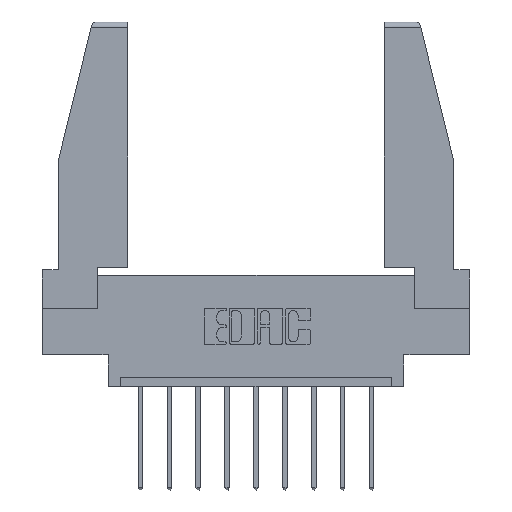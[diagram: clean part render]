
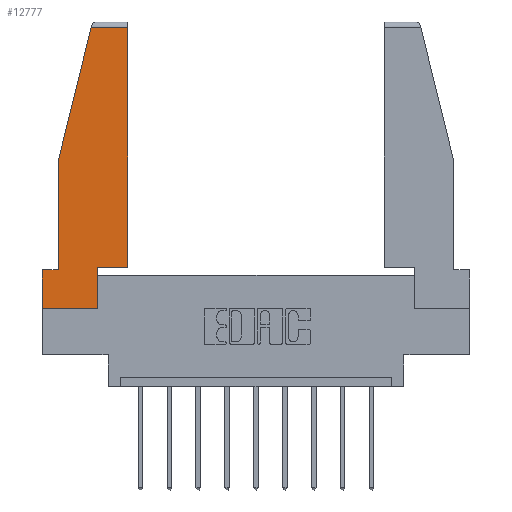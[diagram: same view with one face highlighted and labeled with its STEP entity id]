
A CAD part, top view. The second image highlights one B-rep face of the part: STEP entity #12777.
In plain terms, the highlighted planar face has unit normal (0, 0, 1).
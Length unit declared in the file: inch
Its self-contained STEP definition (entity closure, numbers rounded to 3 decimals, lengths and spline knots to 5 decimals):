
#294 = VECTOR ( 'NONE', #7641, 39.37008 ) ;
#522 = VECTOR ( 'NONE', #7283, 39.37008 ) ;
#584 = VERTEX_POINT ( 'NONE', #11970 ) ;
#839 = CARTESIAN_POINT ( 'NONE',  ( 0., 0.21, 0. ) ) ;
#1178 = DIRECTION ( 'NONE',  ( 1., 0., 0. ) ) ;
#1516 = EDGE_CURVE ( 'NONE', #584, #4535, #6369, .T. ) ;
#1833 = ORIENTED_EDGE ( 'NONE', *, *, #11407, .T. ) ;
#1986 = ORIENTED_EDGE ( 'NONE', *, *, #10798, .T. ) ;
#1992 = EDGE_CURVE ( 'NONE', #4535, #5249, #11923, .T. ) ;
#1998 = CARTESIAN_POINT ( 'NONE',  ( 0.2636, 1.52, 0. ) ) ;
#2097 = EDGE_LOOP ( 'NONE', ( #1986, #8258, #13383, #1833, #10948, #2662, #8005, #8778, #3963 ) ) ;
#2192 = LINE ( 'NONE', #2314, #13155 ) ;
#2307 = LINE ( 'NONE', #11112, #522 ) ;
#2314 = CARTESIAN_POINT ( 'NONE',  ( 0., 0., 0. ) ) ;
#2662 = ORIENTED_EDGE ( 'NONE', *, *, #1992, .T. ) ;
#2899 = VECTOR ( 'NONE', #10846, 39.37008 ) ;
#3237 = EDGE_CURVE ( 'NONE', #8121, #9064, #6634, .T. ) ;
#3409 = EDGE_CURVE ( 'NONE', #4603, #11067, #10568, .T. ) ;
#3734 = VERTEX_POINT ( 'NONE', #4488 ) ;
#3735 = LINE ( 'NONE', #11987, #2899 ) ;
#3963 = ORIENTED_EDGE ( 'NONE', *, *, #3237, .T. ) ;
#4488 = CARTESIAN_POINT ( 'NONE',  ( 0.297, 0., 0. ) ) ;
#4535 = VERTEX_POINT ( 'NONE', #5015 ) ;
#4603 = VERTEX_POINT ( 'NONE', #11184 ) ;
#4656 = DIRECTION ( 'NONE',  ( 0., 0., 1. ) ) ;
#4754 = AXIS2_PLACEMENT_3D ( 'NONE', #4843, #4656, #13100 ) ;
#4843 = CARTESIAN_POINT ( 'NONE',  ( 0., 0., 0. ) ) ;
#5015 = CARTESIAN_POINT ( 'NONE',  ( 0., 0.21, 0. ) ) ;
#5249 = VERTEX_POINT ( 'NONE', #11432 ) ;
#5643 = VECTOR ( 'NONE', #7151, 39.37008 ) ;
#6132 = DIRECTION ( 'NONE',  ( -0.239, -0.971, 0. ) ) ;
#6199 = CARTESIAN_POINT ( 'NONE',  ( 0., 1.52, 0. ) ) ;
#6369 = LINE ( 'NONE', #6606, #294 ) ;
#6569 = FACE_OUTER_BOUND ( 'NONE', #2097, .T. ) ;
#6572 = CARTESIAN_POINT ( 'NONE',  ( 0.297, 0.223, 0. ) ) ;
#6606 = CARTESIAN_POINT ( 'NONE',  ( 0., 0.21, 0. ) ) ;
#6634 = LINE ( 'NONE', #6572, #12538 ) ;
#7151 = DIRECTION ( 'NONE',  ( -1., 0., 0. ) ) ;
#7283 = DIRECTION ( 'NONE',  ( 0., 1., 0. ) ) ;
#7329 = LINE ( 'NONE', #10153, #8468 ) ;
#7605 = DIRECTION ( 'NONE',  ( 1., 0., 0. ) ) ;
#7641 = DIRECTION ( 'NONE',  ( -1., 0., 0. ) ) ;
#7956 = CARTESIAN_POINT ( 'NONE',  ( 0.271, 1.55, 0. ) ) ;
#8005 = ORIENTED_EDGE ( 'NONE', *, *, #8051, .T. ) ;
#8051 = EDGE_CURVE ( 'NONE', #5249, #3734, #2192, .T. ) ;
#8121 = VERTEX_POINT ( 'NONE', #10989 ) ;
#8258 = ORIENTED_EDGE ( 'NONE', *, *, #3409, .T. ) ;
#8391 = VECTOR ( 'NONE', #6132, 39.37008 ) ;
#8468 = VECTOR ( 'NONE', #11212, 39.37008 ) ;
#8670 = EDGE_CURVE ( 'NONE', #11067, #12480, #8713, .T. ) ;
#8713 = LINE ( 'NONE', #7956, #8391 ) ;
#8778 = ORIENTED_EDGE ( 'NONE', *, *, #9384, .T. ) ;
#8870 = PLANE ( 'NONE',  #4754 ) ;
#9064 = VERTEX_POINT ( 'NONE', #9592 ) ;
#9112 = VECTOR ( 'NONE', #11271, 39.37008 ) ;
#9384 = EDGE_CURVE ( 'NONE', #3734, #8121, #2307, .T. ) ;
#9592 = CARTESIAN_POINT ( 'NONE',  ( 0.461, 0.223, 0. ) ) ;
#10153 = CARTESIAN_POINT ( 'NONE',  ( 0.086, 0.8, 0. ) ) ;
#10568 = LINE ( 'NONE', #6199, #5643 ) ;
#10798 = EDGE_CURVE ( 'NONE', #9064, #4603, #3735, .T. ) ;
#10846 = DIRECTION ( 'NONE',  ( 0., 1., 0. ) ) ;
#10948 = ORIENTED_EDGE ( 'NONE', *, *, #1516, .T. ) ;
#10989 = CARTESIAN_POINT ( 'NONE',  ( 0.297, 0.223, 0. ) ) ;
#11067 = VERTEX_POINT ( 'NONE', #1998 ) ;
#11112 = CARTESIAN_POINT ( 'NONE',  ( 0.297, 0., 0. ) ) ;
#11184 = CARTESIAN_POINT ( 'NONE',  ( 0.461, 1.52, 0. ) ) ;
#11212 = DIRECTION ( 'NONE',  ( 0., -1., 0. ) ) ;
#11271 = DIRECTION ( 'NONE',  ( 0., -1., 0. ) ) ;
#11407 = EDGE_CURVE ( 'NONE', #12480, #584, #7329, .T. ) ;
#11432 = CARTESIAN_POINT ( 'NONE',  ( 0., 0., 0. ) ) ;
#11436 = CARTESIAN_POINT ( 'NONE',  ( 0.086, 0.8, 0. ) ) ;
#11923 = LINE ( 'NONE', #839, #9112 ) ;
#11970 = CARTESIAN_POINT ( 'NONE',  ( 0.086, 0.21, 0. ) ) ;
#11987 = CARTESIAN_POINT ( 'NONE',  ( 0.461, 0.223, 0. ) ) ;
#12480 = VERTEX_POINT ( 'NONE', #11436 ) ;
#12538 = VECTOR ( 'NONE', #7605, 39.37008 ) ;
#12777 = ADVANCED_FACE ( 'NONE', ( #6569 ), #8870, .T. ) ;
#13100 = DIRECTION ( 'NONE',  ( 1., 0., 0. ) ) ;
#13155 = VECTOR ( 'NONE', #1178, 39.37008 ) ;
#13383 = ORIENTED_EDGE ( 'NONE', *, *, #8670, .T. ) ;
